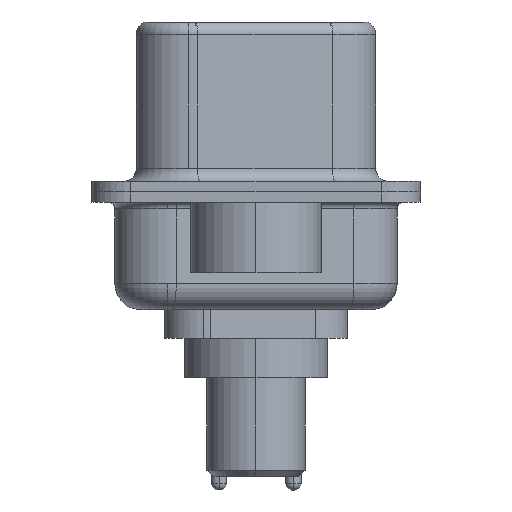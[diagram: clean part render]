
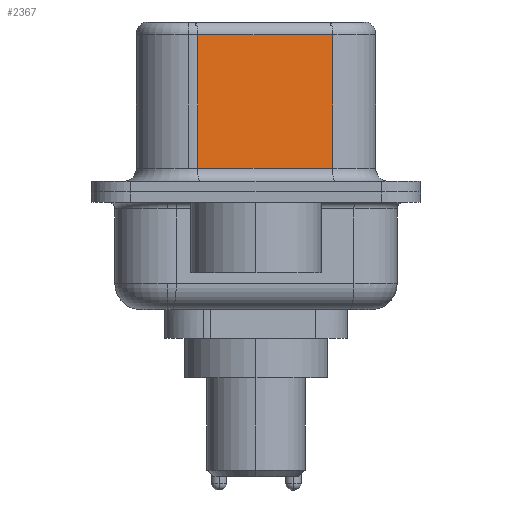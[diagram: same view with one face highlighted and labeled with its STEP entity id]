
A CAD part, left-side view. The second image highlights one B-rep face of the part: STEP entity #2367.
In plain terms, the highlighted planar face has unit normal (-0.985, -0.174, 0).
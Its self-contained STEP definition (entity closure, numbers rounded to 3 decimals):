
#45 = CARTESIAN_POINT ( 'NONE',  ( 4.58, -2.927, 0.9 ) ) ;
#654 = ORIENTED_EDGE ( 'NONE', *, *, #13392, .T. ) ;
#2367 = ADVANCED_FACE ( 'NONE', ( #8861 ), #6895, .F. ) ;
#2512 = ORIENTED_EDGE ( 'NONE', *, *, #10647, .T. ) ;
#2931 = CARTESIAN_POINT ( 'NONE',  ( 3.67, 2.233, 6.52 ) ) ;
#3173 = CARTESIAN_POINT ( 'NONE',  ( 4.58, -2.927, 0.9 ) ) ;
#3608 = EDGE_CURVE ( 'NONE', #11428, #14323, #18185, .T. ) ;
#4477 = ORIENTED_EDGE ( 'NONE', *, *, #18870, .F. ) ;
#4865 = CARTESIAN_POINT ( 'NONE',  ( 4.58, -2.927, 6.02 ) ) ;
#5532 = DIRECTION ( 'NONE',  ( 0., 0., -1. ) ) ;
#6895 = PLANE ( 'NONE',  #14950 ) ;
#6928 = CARTESIAN_POINT ( 'NONE',  ( 3.67, 2.233, 6.02 ) ) ;
#7123 = VERTEX_POINT ( 'NONE', #11676 ) ;
#7571 = LINE ( 'NONE', #45, #10567 ) ;
#8111 = DIRECTION ( 'NONE',  ( -0.174, 0.985, 0. ) ) ;
#8861 = FACE_OUTER_BOUND ( 'NONE', #15357, .T. ) ;
#10567 = VECTOR ( 'NONE', #13319, 1000. ) ;
#10647 = EDGE_CURVE ( 'NONE', #14323, #7123, #15168, .T. ) ;
#10732 = VERTEX_POINT ( 'NONE', #3173 ) ;
#10962 = CARTESIAN_POINT ( 'NONE',  ( 4.58, -2.927, 6.52 ) ) ;
#11428 = VERTEX_POINT ( 'NONE', #14746 ) ;
#11676 = CARTESIAN_POINT ( 'NONE',  ( 3.67, 2.233, 0.9 ) ) ;
#13033 = DIRECTION ( 'NONE',  ( 0.985, 0.174, 0. ) ) ;
#13228 = DIRECTION ( 'NONE',  ( 0., 0., -1. ) ) ;
#13319 = DIRECTION ( 'NONE',  ( 0.174, -0.985, 0. ) ) ;
#13392 = EDGE_CURVE ( 'NONE', #7123, #10732, #7571, .T. ) ;
#14323 = VERTEX_POINT ( 'NONE', #6928 ) ;
#14746 = CARTESIAN_POINT ( 'NONE',  ( 4.58, -2.927, 6.02 ) ) ;
#14950 = AXIS2_PLACEMENT_3D ( 'NONE', #10962, #13033, #8111 ) ;
#15168 = LINE ( 'NONE', #2931, #18662 ) ;
#15357 = EDGE_LOOP ( 'NONE', ( #4477, #18419, #2512, #654 ) ) ;
#15637 = LINE ( 'NONE', #17416, #16119 ) ;
#16119 = VECTOR ( 'NONE', #5532, 1000. ) ;
#16169 = DIRECTION ( 'NONE',  ( -0.174, 0.985, 0. ) ) ;
#17253 = VECTOR ( 'NONE', #16169, 1000. ) ;
#17416 = CARTESIAN_POINT ( 'NONE',  ( 4.58, -2.927, 6.52 ) ) ;
#18185 = LINE ( 'NONE', #4865, #17253 ) ;
#18419 = ORIENTED_EDGE ( 'NONE', *, *, #3608, .T. ) ;
#18662 = VECTOR ( 'NONE', #13228, 1000. ) ;
#18870 = EDGE_CURVE ( 'NONE', #11428, #10732, #15637, .T. ) ;
